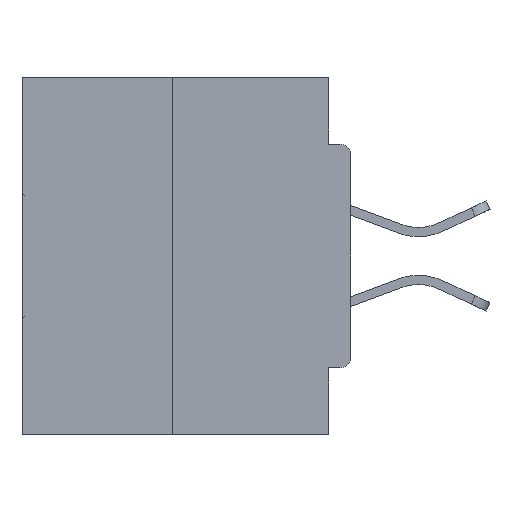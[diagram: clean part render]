
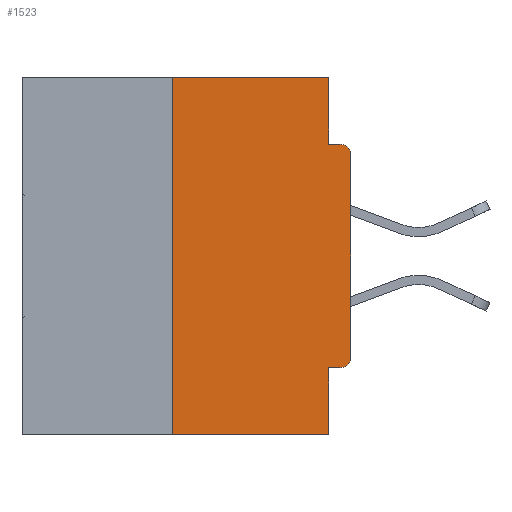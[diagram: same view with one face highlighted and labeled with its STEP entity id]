
A CAD part, left-side view. The second image highlights one B-rep face of the part: STEP entity #1523.
In plain terms, the highlighted planar face has unit normal (-1, 0, 0).
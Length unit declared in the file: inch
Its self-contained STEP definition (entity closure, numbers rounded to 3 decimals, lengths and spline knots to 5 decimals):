
#403 = CARTESIAN_POINT ( 'NONE',  ( 0., 0.015, -0.4065 ) ) ;
#801 = CARTESIAN_POINT ( 'NONE',  ( 0., 0.015, -0.0935 ) ) ;
#1523 = ADVANCED_FACE ( 'NONE', ( #3725 ), #22822, .F. ) ;
#3725 = FACE_OUTER_BOUND ( 'NONE', #40729, .T. ) ;
#3885 = ORIENTED_EDGE ( 'NONE', *, *, #40553, .F. ) ;
#4102 = LINE ( 'NONE', #8333, #11032 ) ;
#4683 = LINE ( 'NONE', #37638, #38674 ) ;
#4860 = CARTESIAN_POINT ( 'NONE',  ( 0., 0.031, 0. ) ) ;
#5268 = CARTESIAN_POINT ( 'NONE',  ( 0., 0., 0. ) ) ;
#6068 = CIRCLE ( 'NONE', #14074, 0.015 ) ;
#6386 = CARTESIAN_POINT ( 'NONE',  ( 0., 0.25, -0.5 ) ) ;
#7885 = CARTESIAN_POINT ( 'NONE',  ( 0., 0.25, 0. ) ) ;
#8333 = CARTESIAN_POINT ( 'NONE',  ( 0., 0.46, -0.5 ) ) ;
#8956 = ORIENTED_EDGE ( 'NONE', *, *, #39451, .T. ) ;
#9723 = VERTEX_POINT ( 'NONE', #11145 ) ;
#10296 = VERTEX_POINT ( 'NONE', #801 ) ;
#10297 = CARTESIAN_POINT ( 'NONE',  ( 0., 0.46, 0. ) ) ;
#10414 = CARTESIAN_POINT ( 'NONE',  ( 0., 0., -0.1085 ) ) ;
#11006 = CARTESIAN_POINT ( 'NONE',  ( 0., 0.031, -0.4065 ) ) ;
#11032 = VECTOR ( 'NONE', #40019, 39.37008 ) ;
#11109 = VERTEX_POINT ( 'NONE', #31979 ) ;
#11145 = CARTESIAN_POINT ( 'NONE',  ( 0., 0.25, 0. ) ) ;
#11279 = VERTEX_POINT ( 'NONE', #18806 ) ;
#12052 = VECTOR ( 'NONE', #22594, 39.37008 ) ;
#12123 = DIRECTION ( 'NONE',  ( 0., 0., -1. ) ) ;
#13467 = DIRECTION ( 'NONE',  ( 1., 0., 0. ) ) ;
#13912 = LINE ( 'NONE', #17202, #16838 ) ;
#14074 = AXIS2_PLACEMENT_3D ( 'NONE', #37184, #34288, #12123 ) ;
#14412 = EDGE_CURVE ( 'NONE', #20618, #10296, #6068, .T. ) ;
#14964 = ORIENTED_EDGE ( 'NONE', *, *, #31320, .F. ) ;
#15203 = LINE ( 'NONE', #5268, #25571 ) ;
#15383 = VERTEX_POINT ( 'NONE', #11006 ) ;
#16838 = VECTOR ( 'NONE', #22998, 39.37008 ) ;
#17202 = CARTESIAN_POINT ( 'NONE',  ( 0., 0.031, -0.5 ) ) ;
#17841 = VERTEX_POINT ( 'NONE', #18695 ) ;
#18423 = VERTEX_POINT ( 'NONE', #403 ) ;
#18695 = CARTESIAN_POINT ( 'NONE',  ( 0., 0.031, 0. ) ) ;
#18806 = CARTESIAN_POINT ( 'NONE',  ( 0., 0.031, -0.5 ) ) ;
#18946 = ORIENTED_EDGE ( 'NONE', *, *, #21049, .F. ) ;
#19208 = CARTESIAN_POINT ( 'NONE',  ( 0., 0., -0.4065 ) ) ;
#19273 = CARTESIAN_POINT ( 'NONE',  ( 0., 0.46, 0. ) ) ;
#19275 = VECTOR ( 'NONE', #27307, 39.37008 ) ;
#20618 = VERTEX_POINT ( 'NONE', #10414 ) ;
#21034 = EDGE_CURVE ( 'NONE', #35098, #10296, #4683, .T. ) ;
#21049 = EDGE_CURVE ( 'NONE', #9723, #17841, #23885, .T. ) ;
#22402 = VECTOR ( 'NONE', #39743, 39.37008 ) ;
#22465 = DIRECTION ( 'NONE',  ( 0., -1., 0. ) ) ;
#22594 = DIRECTION ( 'NONE',  ( 0., -1., 0. ) ) ;
#22612 = DIRECTION ( 'NONE',  ( -1., 0., 0. ) ) ;
#22822 = PLANE ( 'NONE',  #31151 ) ;
#22998 = DIRECTION ( 'NONE',  ( 0., 0., -1. ) ) ;
#23264 = LINE ( 'NONE', #4860, #19275 ) ;
#23885 = LINE ( 'NONE', #19273, #12052 ) ;
#24092 = VECTOR ( 'NONE', #38121, 39.37008 ) ;
#24870 = EDGE_CURVE ( 'NONE', #11109, #20618, #15203, .T. ) ;
#25098 = ORIENTED_EDGE ( 'NONE', *, *, #33484, .T. ) ;
#25571 = VECTOR ( 'NONE', #33097, 39.37008 ) ;
#25928 = DIRECTION ( 'NONE',  ( 0., 0., -1. ) ) ;
#26191 = ORIENTED_EDGE ( 'NONE', *, *, #24870, .T. ) ;
#27307 = DIRECTION ( 'NONE',  ( 0., 0., -1. ) ) ;
#29001 = LINE ( 'NONE', #19208, #24092 ) ;
#31151 = AXIS2_PLACEMENT_3D ( 'NONE', #10297, #13467, #36189 ) ;
#31320 = EDGE_CURVE ( 'NONE', #17841, #35098, #23264, .T. ) ;
#31676 = ORIENTED_EDGE ( 'NONE', *, *, #35957, .F. ) ;
#31979 = CARTESIAN_POINT ( 'NONE',  ( 0., 0., -0.3915 ) ) ;
#32478 = AXIS2_PLACEMENT_3D ( 'NONE', #35424, #22612, #25928 ) ;
#32709 = EDGE_CURVE ( 'NONE', #37815, #9723, #38192, .T. ) ;
#33097 = DIRECTION ( 'NONE',  ( 0., 0., 1. ) ) ;
#33484 = EDGE_CURVE ( 'NONE', #18423, #11109, #34659, .T. ) ;
#34288 = DIRECTION ( 'NONE',  ( -1., 0., 0. ) ) ;
#34659 = CIRCLE ( 'NONE', #32478, 0.015 ) ;
#35098 = VERTEX_POINT ( 'NONE', #35427 ) ;
#35424 = CARTESIAN_POINT ( 'NONE',  ( 0., 0.015, -0.3915 ) ) ;
#35427 = CARTESIAN_POINT ( 'NONE',  ( 0., 0.031, -0.0935 ) ) ;
#35957 = EDGE_CURVE ( 'NONE', #18423, #15383, #29001, .T. ) ;
#36189 = DIRECTION ( 'NONE',  ( 0., 0., -1. ) ) ;
#37184 = CARTESIAN_POINT ( 'NONE',  ( 0., 0.015, -0.1085 ) ) ;
#37638 = CARTESIAN_POINT ( 'NONE',  ( 0., 0., -0.0935 ) ) ;
#37815 = VERTEX_POINT ( 'NONE', #6386 ) ;
#38070 = ORIENTED_EDGE ( 'NONE', *, *, #14412, .T. ) ;
#38121 = DIRECTION ( 'NONE',  ( 0., 1., 0. ) ) ;
#38192 = LINE ( 'NONE', #7885, #22402 ) ;
#38674 = VECTOR ( 'NONE', #22465, 39.37008 ) ;
#38973 = ORIENTED_EDGE ( 'NONE', *, *, #32709, .F. ) ;
#39451 = EDGE_CURVE ( 'NONE', #37815, #11279, #4102, .T. ) ;
#39743 = DIRECTION ( 'NONE',  ( 0., 0., 1. ) ) ;
#40019 = DIRECTION ( 'NONE',  ( 0., -1., 0. ) ) ;
#40092 = ORIENTED_EDGE ( 'NONE', *, *, #21034, .F. ) ;
#40553 = EDGE_CURVE ( 'NONE', #15383, #11279, #13912, .T. ) ;
#40729 = EDGE_LOOP ( 'NONE', ( #18946, #38973, #8956, #3885, #31676, #25098, #26191, #38070, #40092, #14964 ) ) ;
